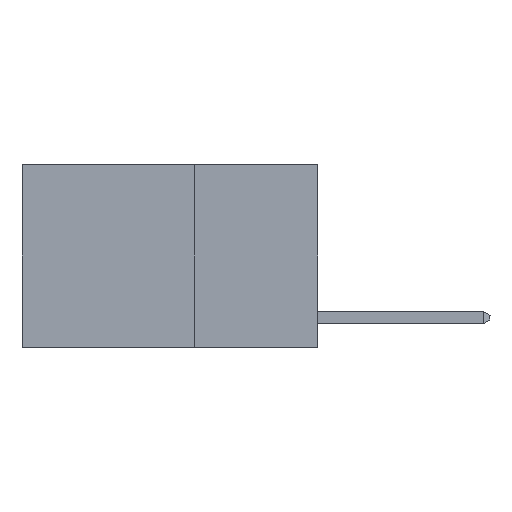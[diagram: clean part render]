
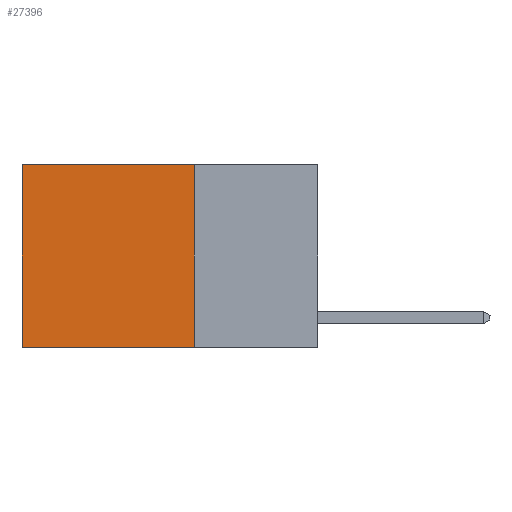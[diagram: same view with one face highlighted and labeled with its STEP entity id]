
A CAD part, left-side view. The second image highlights one B-rep face of the part: STEP entity #27396.
In plain terms, the highlighted planar face has unit normal (-1, 0, 0).
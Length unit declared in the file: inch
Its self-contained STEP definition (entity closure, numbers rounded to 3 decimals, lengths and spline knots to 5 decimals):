
#1684 = CARTESIAN_POINT ( 'NONE',  ( 0.2625, 0.25, -0.37 ) ) ;
#4138 = EDGE_CURVE ( 'NONE', #8169, #24937, #11091, .T. ) ;
#4513 = ORIENTED_EDGE ( 'NONE', *, *, #7316, .T. ) ;
#4612 = VECTOR ( 'NONE', #8411, 39.37008 ) ;
#5287 = DIRECTION ( 'NONE',  ( 0., 0., -1. ) ) ;
#5648 = VECTOR ( 'NONE', #5287, 39.37008 ) ;
#6304 = PLANE ( 'NONE',  #12915 ) ;
#6642 = CARTESIAN_POINT ( 'NONE',  ( 0.2625, 0.6, 0. ) ) ;
#6651 = CARTESIAN_POINT ( 'NONE',  ( 0.2625, 0.25, 0. ) ) ;
#7316 = EDGE_CURVE ( 'NONE', #8169, #17460, #24771, .T. ) ;
#8169 = VERTEX_POINT ( 'NONE', #6651 ) ;
#8411 = DIRECTION ( 'NONE',  ( 0., 1., 0. ) ) ;
#8636 = DIRECTION ( 'NONE',  ( 1., 0., 0. ) ) ;
#9826 = CARTESIAN_POINT ( 'NONE',  ( 0.2625, 0.6, -0.37 ) ) ;
#9962 = VECTOR ( 'NONE', #29306, 39.37008 ) ;
#10767 = LINE ( 'NONE', #28760, #4612 ) ;
#11091 = LINE ( 'NONE', #19069, #5648 ) ;
#12915 = AXIS2_PLACEMENT_3D ( 'NONE', #13200, #8636, #24600 ) ;
#13200 = CARTESIAN_POINT ( 'NONE',  ( 0.2625, 0.25, 0. ) ) ;
#13234 = ORIENTED_EDGE ( 'NONE', *, *, #27996, .F. ) ;
#13686 = DIRECTION ( 'NONE',  ( 0., 1., 0. ) ) ;
#16221 = EDGE_CURVE ( 'NONE', #17460, #17833, #16809, .T. ) ;
#16384 = EDGE_LOOP ( 'NONE', ( #28311, #13234, #19066, #4513 ) ) ;
#16809 = LINE ( 'NONE', #6642, #9962 ) ;
#17460 = VERTEX_POINT ( 'NONE', #19860 ) ;
#17833 = VERTEX_POINT ( 'NONE', #9826 ) ;
#19066 = ORIENTED_EDGE ( 'NONE', *, *, #4138, .F. ) ;
#19069 = CARTESIAN_POINT ( 'NONE',  ( 0.2625, 0.25, 0. ) ) ;
#19860 = CARTESIAN_POINT ( 'NONE',  ( 0.2625, 0.6, 0. ) ) ;
#24600 = DIRECTION ( 'NONE',  ( 0., 0., -1. ) ) ;
#24771 = LINE ( 'NONE', #29557, #25487 ) ;
#24937 = VERTEX_POINT ( 'NONE', #1684 ) ;
#25487 = VECTOR ( 'NONE', #13686, 39.37008 ) ;
#27396 = ADVANCED_FACE ( 'NONE', ( #27865 ), #6304, .F. ) ;
#27865 = FACE_OUTER_BOUND ( 'NONE', #16384, .T. ) ;
#27996 = EDGE_CURVE ( 'NONE', #24937, #17833, #10767, .T. ) ;
#28311 = ORIENTED_EDGE ( 'NONE', *, *, #16221, .T. ) ;
#28760 = CARTESIAN_POINT ( 'NONE',  ( 0.2625, 0.25, -0.37 ) ) ;
#29306 = DIRECTION ( 'NONE',  ( 0., 0., -1. ) ) ;
#29557 = CARTESIAN_POINT ( 'NONE',  ( 0.2625, 0.25, 0. ) ) ;
